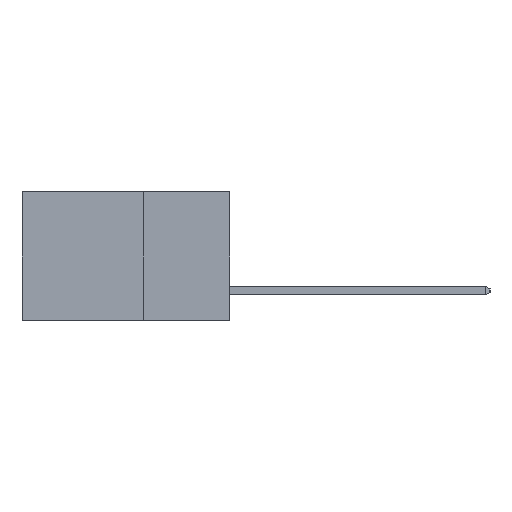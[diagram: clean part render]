
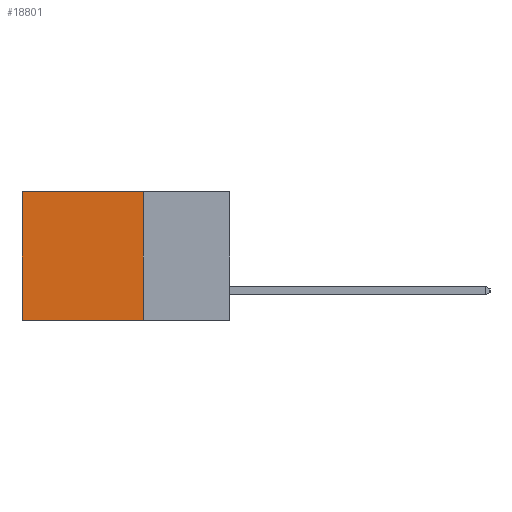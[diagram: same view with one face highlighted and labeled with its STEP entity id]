
A CAD part, left-side view. The second image highlights one B-rep face of the part: STEP entity #18801.
In plain terms, the highlighted planar face has unit normal (-1, 0, 0).
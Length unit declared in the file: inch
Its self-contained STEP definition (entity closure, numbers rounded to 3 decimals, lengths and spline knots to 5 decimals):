
#458 = DIRECTION ( 'NONE',  ( 0., 1., 0. ) ) ;
#697 = CARTESIAN_POINT ( 'NONE',  ( 0.2615, 0.25, -0.37 ) ) ;
#2650 = DIRECTION ( 'NONE',  ( 0., 0., -1. ) ) ;
#3267 = FACE_OUTER_BOUND ( 'NONE', #21062, .T. ) ;
#3825 = LINE ( 'NONE', #10800, #8373 ) ;
#3866 = VERTEX_POINT ( 'NONE', #17406 ) ;
#4372 = LINE ( 'NONE', #12032, #14618 ) ;
#4394 = CARTESIAN_POINT ( 'NONE',  ( 0.2615, 0.25, -0.37 ) ) ;
#4522 = CARTESIAN_POINT ( 'NONE',  ( 0.2615, 0.25, -0.37 ) ) ;
#4699 = CARTESIAN_POINT ( 'NONE',  ( 0.2615, 0.25, -0.37 ) ) ;
#4818 = LINE ( 'NONE', #4394, #24474 ) ;
#6047 = VERTEX_POINT ( 'NONE', #7019 ) ;
#6545 = VERTEX_POINT ( 'NONE', #4522 ) ;
#6900 = DIRECTION ( 'NONE',  ( 0., 0., -1. ) ) ;
#7019 = CARTESIAN_POINT ( 'NONE',  ( 0.2615, 0.6, 0. ) ) ;
#7363 = ORIENTED_EDGE ( 'NONE', *, *, #22674, .F. ) ;
#8373 = VECTOR ( 'NONE', #6900, 39.37008 ) ;
#10207 = VERTEX_POINT ( 'NONE', #18708 ) ;
#10552 = ORIENTED_EDGE ( 'NONE', *, *, #19614, .T. ) ;
#10800 = CARTESIAN_POINT ( 'NONE',  ( 0.2615, 0.6, -0.37 ) ) ;
#12032 = CARTESIAN_POINT ( 'NONE',  ( 0.2615, 0.25, 0. ) ) ;
#12156 = DIRECTION ( 'NONE',  ( 0., 1., 0. ) ) ;
#12250 = PLANE ( 'NONE',  #15545 ) ;
#13896 = ORIENTED_EDGE ( 'NONE', *, *, #19507, .F. ) ;
#14184 = DIRECTION ( 'NONE',  ( 1., 0., 0. ) ) ;
#14618 = VECTOR ( 'NONE', #458, 39.37008 ) ;
#15545 = AXIS2_PLACEMENT_3D ( 'NONE', #697, #14184, #2650 ) ;
#15904 = VECTOR ( 'NONE', #18178, 39.37008 ) ;
#16290 = ORIENTED_EDGE ( 'NONE', *, *, #16379, .T. ) ;
#16379 = EDGE_CURVE ( 'NONE', #3866, #6047, #4372, .T. ) ;
#17406 = CARTESIAN_POINT ( 'NONE',  ( 0.2615, 0.25, 0. ) ) ;
#18178 = DIRECTION ( 'NONE',  ( 0., 0., -1. ) ) ;
#18708 = CARTESIAN_POINT ( 'NONE',  ( 0.2615, 0.6, -0.37 ) ) ;
#18801 = ADVANCED_FACE ( 'NONE', ( #3267 ), #12250, .F. ) ;
#19507 = EDGE_CURVE ( 'NONE', #3866, #6545, #22082, .T. ) ;
#19614 = EDGE_CURVE ( 'NONE', #6047, #10207, #3825, .T. ) ;
#21062 = EDGE_LOOP ( 'NONE', ( #10552, #7363, #13896, #16290 ) ) ;
#22082 = LINE ( 'NONE', #4699, #15904 ) ;
#22674 = EDGE_CURVE ( 'NONE', #6545, #10207, #4818, .T. ) ;
#24474 = VECTOR ( 'NONE', #12156, 39.37008 ) ;
